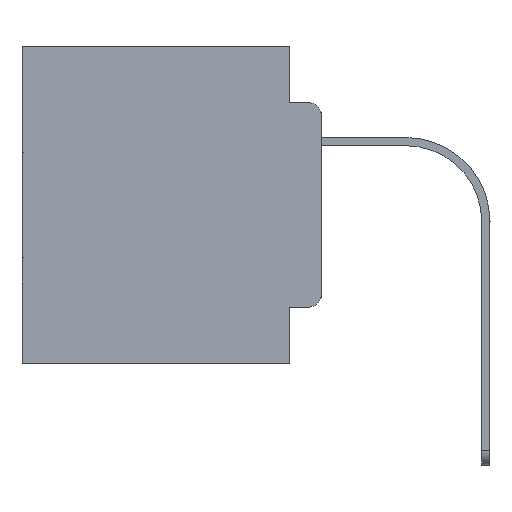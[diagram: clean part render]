
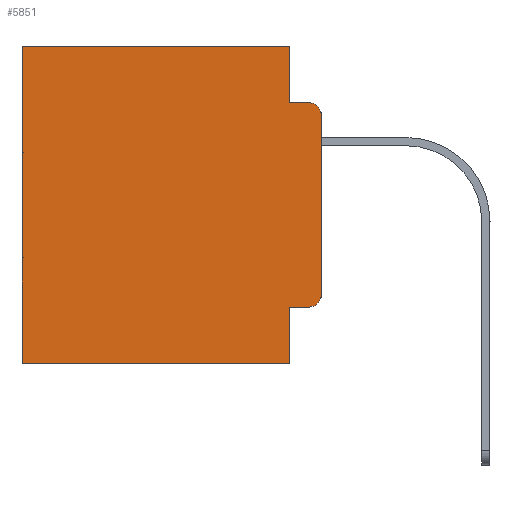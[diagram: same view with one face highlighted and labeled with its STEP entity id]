
A CAD part, left-side view. The second image highlights one B-rep face of the part: STEP entity #5851.
In plain terms, the highlighted planar face has unit normal (-1, 0, 0).
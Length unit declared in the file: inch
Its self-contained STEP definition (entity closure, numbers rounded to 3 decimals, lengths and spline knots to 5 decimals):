
#88 = DIRECTION ( 'NONE',  ( 0., 0., -1. ) ) ;
#630 = PLANE ( 'NONE',  #6220 ) ;
#638 = EDGE_CURVE ( 'NONE', #27244, #18021, #16178, .T. ) ;
#922 = EDGE_CURVE ( 'NONE', #21604, #20832, #1646, .T. ) ;
#1335 = CARTESIAN_POINT ( 'NONE',  ( 0.298, 0., -0.5 ) ) ;
#1541 = CARTESIAN_POINT ( 'NONE',  ( 0.298, 0.473, 0. ) ) ;
#1646 = LINE ( 'NONE', #1335, #23679 ) ;
#1789 = CARTESIAN_POINT ( 'NONE',  ( 0.298, 0.051, -0.0885 ) ) ;
#1852 = CARTESIAN_POINT ( 'NONE',  ( 0.298, 0.473, 0. ) ) ;
#1926 = VECTOR ( 'NONE', #8635, 39.37008 ) ;
#2211 = VERTEX_POINT ( 'NONE', #1789 ) ;
#3234 = EDGE_CURVE ( 'NONE', #17869, #21604, #9411, .T. ) ;
#3341 = CARTESIAN_POINT ( 'NONE',  ( 0.298, 0.473, -0.5 ) ) ;
#3788 = EDGE_LOOP ( 'NONE', ( #19309, #18524, #24260, #19062, #5399, #3932, #17591, #22537, #14591, #28109 ) ) ;
#3932 = ORIENTED_EDGE ( 'NONE', *, *, #22325, .T. ) ;
#4921 = CARTESIAN_POINT ( 'NONE',  ( 0.298, 0.02, -0.1085 ) ) ;
#5003 = CARTESIAN_POINT ( 'NONE',  ( 0.298, 0.051, -0.5 ) ) ;
#5399 = ORIENTED_EDGE ( 'NONE', *, *, #24172, .T. ) ;
#5447 = VERTEX_POINT ( 'NONE', #15225 ) ;
#5739 = DIRECTION ( 'NONE',  ( 0., 0., -1. ) ) ;
#5851 = ADVANCED_FACE ( 'NONE', ( #10231 ), #630, .F. ) ;
#5937 = CARTESIAN_POINT ( 'NONE',  ( 0.298, 0., -0.1085 ) ) ;
#5943 = DIRECTION ( 'NONE',  ( 0., -1., 0. ) ) ;
#6220 = AXIS2_PLACEMENT_3D ( 'NONE', #21896, #27178, #5739 ) ;
#6976 = DIRECTION ( 'NONE',  ( 0., 0., -1. ) ) ;
#7054 = LINE ( 'NONE', #23528, #14344 ) ;
#7079 = CARTESIAN_POINT ( 'NONE',  ( 0.298, 0.051, 0. ) ) ;
#8260 = CARTESIAN_POINT ( 'NONE',  ( 0.298, 0.051, -0.4115 ) ) ;
#8430 = VECTOR ( 'NONE', #88, 39.37008 ) ;
#8635 = DIRECTION ( 'NONE',  ( 0., -1., 0. ) ) ;
#9411 = LINE ( 'NONE', #7079, #17661 ) ;
#10231 = FACE_OUTER_BOUND ( 'NONE', #3788, .T. ) ;
#10759 = CARTESIAN_POINT ( 'NONE',  ( 0.298, 0.051, -0.4115 ) ) ;
#10958 = CARTESIAN_POINT ( 'NONE',  ( 0.298, 0.051, -0.0885 ) ) ;
#11215 = AXIS2_PLACEMENT_3D ( 'NONE', #4921, #16404, #23406 ) ;
#13110 = DIRECTION ( 'NONE',  ( 0., 1., 0. ) ) ;
#13788 = VECTOR ( 'NONE', #21685, 39.37008 ) ;
#13853 = CARTESIAN_POINT ( 'NONE',  ( 0.298, 0.02, -0.0885 ) ) ;
#14320 = EDGE_CURVE ( 'NONE', #27244, #29031, #19091, .T. ) ;
#14344 = VECTOR ( 'NONE', #19317, 39.37008 ) ;
#14591 = ORIENTED_EDGE ( 'NONE', *, *, #29128, .T. ) ;
#14794 = EDGE_CURVE ( 'NONE', #5447, #2211, #26051, .T. ) ;
#15225 = CARTESIAN_POINT ( 'NONE',  ( 0.298, 0.051, 0. ) ) ;
#15640 = LINE ( 'NONE', #1541, #8430 ) ;
#16132 = CARTESIAN_POINT ( 'NONE',  ( 0.298, 0., -0.3915 ) ) ;
#16178 = CIRCLE ( 'NONE', #11215, 0.02 ) ;
#16329 = EDGE_CURVE ( 'NONE', #2211, #18021, #22779, .T. ) ;
#16404 = DIRECTION ( 'NONE',  ( -1., 0., 0. ) ) ;
#16463 = AXIS2_PLACEMENT_3D ( 'NONE', #20296, #24822, #22494 ) ;
#17591 = ORIENTED_EDGE ( 'NONE', *, *, #922, .F. ) ;
#17661 = VECTOR ( 'NONE', #26038, 39.37008 ) ;
#17869 = VERTEX_POINT ( 'NONE', #10759 ) ;
#18021 = VERTEX_POINT ( 'NONE', #13853 ) ;
#18524 = ORIENTED_EDGE ( 'NONE', *, *, #638, .T. ) ;
#18710 = VERTEX_POINT ( 'NONE', #24694 ) ;
#19062 = ORIENTED_EDGE ( 'NONE', *, *, #14794, .F. ) ;
#19091 = LINE ( 'NONE', #26253, #19225 ) ;
#19225 = VECTOR ( 'NONE', #6976, 39.37008 ) ;
#19309 = ORIENTED_EDGE ( 'NONE', *, *, #14320, .F. ) ;
#19317 = DIRECTION ( 'NONE',  ( 0., 1., 0. ) ) ;
#20066 = LINE ( 'NONE', #8260, #20999 ) ;
#20296 = CARTESIAN_POINT ( 'NONE',  ( 0.298, 0.02, -0.3915 ) ) ;
#20832 = VERTEX_POINT ( 'NONE', #3341 ) ;
#20999 = VECTOR ( 'NONE', #5943, 39.37008 ) ;
#21546 = CARTESIAN_POINT ( 'NONE',  ( 0.298, 0.051, 0. ) ) ;
#21604 = VERTEX_POINT ( 'NONE', #5003 ) ;
#21685 = DIRECTION ( 'NONE',  ( 0., 0., -1. ) ) ;
#21896 = CARTESIAN_POINT ( 'NONE',  ( 0.298, 0., 0. ) ) ;
#22325 = EDGE_CURVE ( 'NONE', #24861, #20832, #15640, .T. ) ;
#22494 = DIRECTION ( 'NONE',  ( 0., 0., -1. ) ) ;
#22537 = ORIENTED_EDGE ( 'NONE', *, *, #3234, .F. ) ;
#22779 = LINE ( 'NONE', #10958, #1926 ) ;
#23406 = DIRECTION ( 'NONE',  ( 0., 0., -1. ) ) ;
#23528 = CARTESIAN_POINT ( 'NONE',  ( 0.298, 0., 0. ) ) ;
#23679 = VECTOR ( 'NONE', #13110, 39.37008 ) ;
#24172 = EDGE_CURVE ( 'NONE', #5447, #24861, #7054, .T. ) ;
#24260 = ORIENTED_EDGE ( 'NONE', *, *, #16329, .F. ) ;
#24694 = CARTESIAN_POINT ( 'NONE',  ( 0.298, 0.02, -0.4115 ) ) ;
#24822 = DIRECTION ( 'NONE',  ( -1., 0., 0. ) ) ;
#24861 = VERTEX_POINT ( 'NONE', #1852 ) ;
#26038 = DIRECTION ( 'NONE',  ( 0., 0., -1. ) ) ;
#26051 = LINE ( 'NONE', #21546, #13788 ) ;
#26253 = CARTESIAN_POINT ( 'NONE',  ( 0.298, 0., 0. ) ) ;
#27178 = DIRECTION ( 'NONE',  ( 1., 0., 0. ) ) ;
#27244 = VERTEX_POINT ( 'NONE', #5937 ) ;
#28109 = ORIENTED_EDGE ( 'NONE', *, *, #28340, .T. ) ;
#28340 = EDGE_CURVE ( 'NONE', #18710, #29031, #28862, .T. ) ;
#28862 = CIRCLE ( 'NONE', #16463, 0.02 ) ;
#29031 = VERTEX_POINT ( 'NONE', #16132 ) ;
#29128 = EDGE_CURVE ( 'NONE', #17869, #18710, #20066, .T. ) ;
